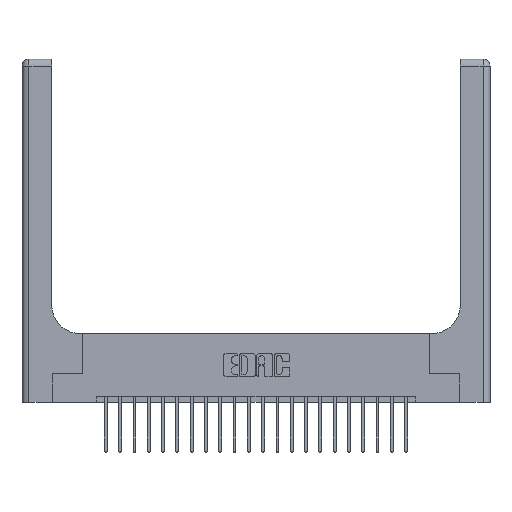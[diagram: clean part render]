
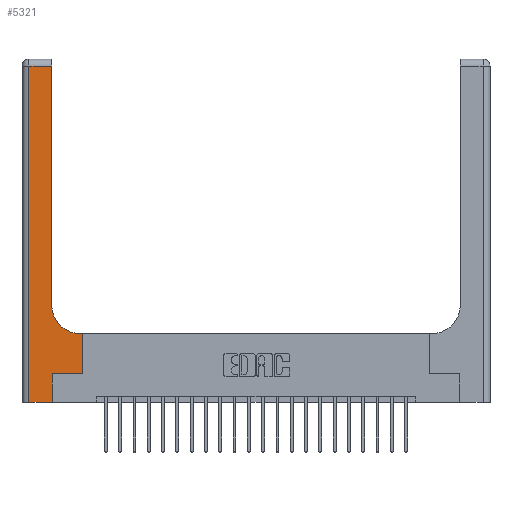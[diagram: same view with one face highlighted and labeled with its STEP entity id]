
A CAD part, top view. The second image highlights one B-rep face of the part: STEP entity #5321.
In plain terms, the highlighted planar face has unit normal (0, 0, 1).
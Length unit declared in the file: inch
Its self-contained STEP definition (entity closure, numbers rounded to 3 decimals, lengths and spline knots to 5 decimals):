
#911 = LINE ( 'NONE', #4473, #13842 ) ;
#1134 = DIRECTION ( 'NONE',  ( 0., 1., 0. ) ) ;
#1586 = DIRECTION ( 'NONE',  ( -1., 0., 0. ) ) ;
#1680 = ORIENTED_EDGE ( 'NONE', *, *, #5889, .T. ) ;
#1900 = DIRECTION ( 'NONE',  ( 1., 0., 0. ) ) ;
#2175 = CIRCLE ( 'NONE', #4357, 0.25 ) ;
#2279 = VERTEX_POINT ( 'NONE', #21204 ) ;
#2311 = DIRECTION ( 'NONE',  ( 0., 0., -1. ) ) ;
#2440 = VECTOR ( 'NONE', #18637, 39.37008 ) ;
#2566 = CARTESIAN_POINT ( 'NONE',  ( 0.26, 2.94, 0.37 ) ) ;
#2825 = DIRECTION ( 'NONE',  ( -1., 0., 0. ) ) ;
#2929 = AXIS2_PLACEMENT_3D ( 'NONE', #21568, #2311, #9706 ) ;
#3034 = CARTESIAN_POINT ( 'NONE',  ( 0.265, 0., 0.37 ) ) ;
#4357 = AXIS2_PLACEMENT_3D ( 'NONE', #11207, #9815, #13137 ) ;
#4473 = CARTESIAN_POINT ( 'NONE',  ( 0.528, 0.25, 0.37 ) ) ;
#4989 = LINE ( 'NONE', #3034, #2440 ) ;
#5257 = LINE ( 'NONE', #8447, #17292 ) ;
#5321 = ADVANCED_FACE ( 'NONE', ( #9265 ), #11432, .F. ) ;
#5356 = LINE ( 'NONE', #12297, #7106 ) ;
#5452 = EDGE_CURVE ( 'NONE', #17005, #20146, #8568, .T. ) ;
#5654 = ORIENTED_EDGE ( 'NONE', *, *, #14553, .T. ) ;
#5889 = EDGE_CURVE ( 'NONE', #7356, #15402, #18880, .T. ) ;
#5916 = VECTOR ( 'NONE', #21008, 39.37008 ) ;
#6630 = EDGE_CURVE ( 'NONE', #15402, #17005, #2175, .T. ) ;
#6727 = EDGE_CURVE ( 'NONE', #2279, #7356, #911, .T. ) ;
#6752 = LINE ( 'NONE', #8698, #5916 ) ;
#7106 = VECTOR ( 'NONE', #10586, 39.37008 ) ;
#7356 = VERTEX_POINT ( 'NONE', #19336 ) ;
#7402 = VECTOR ( 'NONE', #1900, 39.37008 ) ;
#7584 = EDGE_CURVE ( 'NONE', #10861, #17521, #4989, .T. ) ;
#8207 = CARTESIAN_POINT ( 'NONE',  ( 0.26, 0.6, 0.37 ) ) ;
#8447 = CARTESIAN_POINT ( 'NONE',  ( 0., 2.94, 0.37 ) ) ;
#8483 = EDGE_CURVE ( 'NONE', #17521, #2279, #5356, .T. ) ;
#8568 = LINE ( 'NONE', #13697, #21977 ) ;
#8698 = CARTESIAN_POINT ( 'NONE',  ( 0.06, 3., 0.37 ) ) ;
#9265 = FACE_OUTER_BOUND ( 'NONE', #14035, .T. ) ;
#9567 = VERTEX_POINT ( 'NONE', #14377 ) ;
#9706 = DIRECTION ( 'NONE',  ( -1., 0., 0. ) ) ;
#9711 = DIRECTION ( 'NONE',  ( 0., 1., 0. ) ) ;
#9815 = DIRECTION ( 'NONE',  ( 0., 0., -1. ) ) ;
#10220 = LINE ( 'NONE', #10335, #7402 ) ;
#10335 = CARTESIAN_POINT ( 'NONE',  ( 0., 0., 0.37 ) ) ;
#10586 = DIRECTION ( 'NONE',  ( 1., 0., 0. ) ) ;
#10861 = VERTEX_POINT ( 'NONE', #13814 ) ;
#11207 = CARTESIAN_POINT ( 'NONE',  ( 0.51, 0.85, 0.37 ) ) ;
#11432 = PLANE ( 'NONE',  #2929 ) ;
#11691 = ORIENTED_EDGE ( 'NONE', *, *, #8483, .T. ) ;
#12297 = CARTESIAN_POINT ( 'NONE',  ( 0.265, 0.25, 0.37 ) ) ;
#12341 = ORIENTED_EDGE ( 'NONE', *, *, #6630, .T. ) ;
#12990 = CARTESIAN_POINT ( 'NONE',  ( 0.26, 0.85, 0.37 ) ) ;
#13137 = DIRECTION ( 'NONE',  ( 1., 0., 0. ) ) ;
#13697 = CARTESIAN_POINT ( 'NONE',  ( 0.26, 3., 0.37 ) ) ;
#13776 = ORIENTED_EDGE ( 'NONE', *, *, #6727, .T. ) ;
#13814 = CARTESIAN_POINT ( 'NONE',  ( 0.265, 0., 0.37 ) ) ;
#13842 = VECTOR ( 'NONE', #9711, 39.37008 ) ;
#14011 = EDGE_CURVE ( 'NONE', #21671, #9567, #6752, .T. ) ;
#14035 = EDGE_LOOP ( 'NONE', ( #14085, #5654, #15429, #14492, #15993, #11691, #13776, #1680, #12341 ) ) ;
#14085 = ORIENTED_EDGE ( 'NONE', *, *, #5452, .T. ) ;
#14161 = CARTESIAN_POINT ( 'NONE',  ( 0.51, 0.6, 0.37 ) ) ;
#14377 = CARTESIAN_POINT ( 'NONE',  ( 0.06, 0., 0.37 ) ) ;
#14492 = ORIENTED_EDGE ( 'NONE', *, *, #15089, .T. ) ;
#14553 = EDGE_CURVE ( 'NONE', #20146, #21671, #5257, .T. ) ;
#15089 = EDGE_CURVE ( 'NONE', #9567, #10861, #10220, .T. ) ;
#15383 = VECTOR ( 'NONE', #2825, 39.37008 ) ;
#15402 = VERTEX_POINT ( 'NONE', #14161 ) ;
#15429 = ORIENTED_EDGE ( 'NONE', *, *, #14011, .T. ) ;
#15993 = ORIENTED_EDGE ( 'NONE', *, *, #7584, .T. ) ;
#17005 = VERTEX_POINT ( 'NONE', #12990 ) ;
#17292 = VECTOR ( 'NONE', #1586, 39.37008 ) ;
#17521 = VERTEX_POINT ( 'NONE', #21571 ) ;
#18637 = DIRECTION ( 'NONE',  ( 0., 1., 0. ) ) ;
#18753 = CARTESIAN_POINT ( 'NONE',  ( 0.06, 2.94, 0.37 ) ) ;
#18880 = LINE ( 'NONE', #8207, #15383 ) ;
#19336 = CARTESIAN_POINT ( 'NONE',  ( 0.528, 0.6, 0.37 ) ) ;
#20146 = VERTEX_POINT ( 'NONE', #2566 ) ;
#21008 = DIRECTION ( 'NONE',  ( 0., -1., 0. ) ) ;
#21204 = CARTESIAN_POINT ( 'NONE',  ( 0.528, 0.25, 0.37 ) ) ;
#21568 = CARTESIAN_POINT ( 'NONE',  ( 0., 3., 0.37 ) ) ;
#21571 = CARTESIAN_POINT ( 'NONE',  ( 0.265, 0.25, 0.37 ) ) ;
#21671 = VERTEX_POINT ( 'NONE', #18753 ) ;
#21977 = VECTOR ( 'NONE', #1134, 39.37008 ) ;
